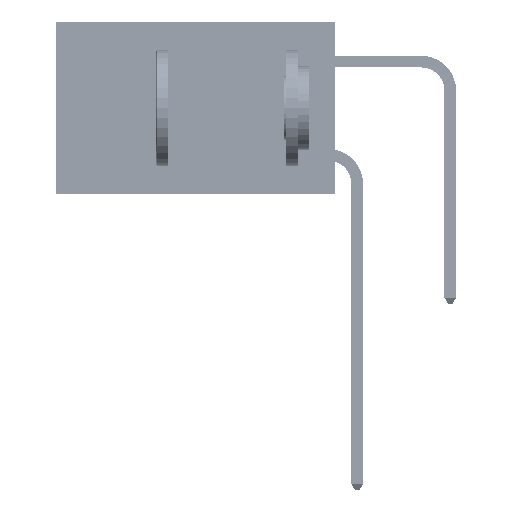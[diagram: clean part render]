
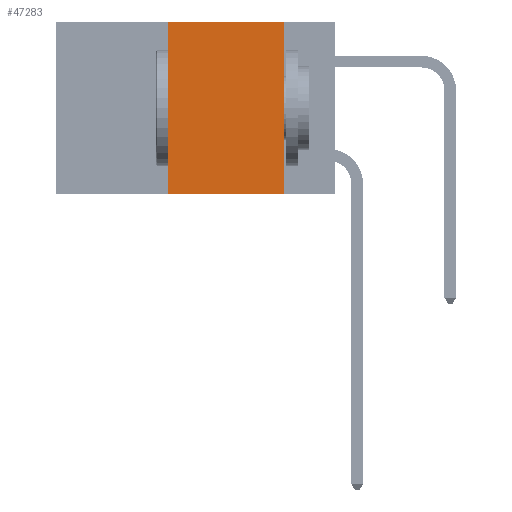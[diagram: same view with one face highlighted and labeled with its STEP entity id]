
A CAD part, left-side view. The second image highlights one B-rep face of the part: STEP entity #47283.
In plain terms, the highlighted planar face has unit normal (-1, 0, 0).
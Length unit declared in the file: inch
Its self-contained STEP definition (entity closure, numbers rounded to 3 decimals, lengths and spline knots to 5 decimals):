
#4005 = DIRECTION ( 'NONE',  ( 0., 0., -1. ) ) ;
#4142 = EDGE_CURVE ( 'NONE', #15398, #4536, #16195, .T. ) ;
#4536 = VERTEX_POINT ( 'NONE', #39910 ) ;
#6880 = ORIENTED_EDGE ( 'NONE', *, *, #33889, .F. ) ;
#7804 = LINE ( 'NONE', #27506, #16931 ) ;
#8382 = EDGE_CURVE ( 'NONE', #39591, #4536, #23125, .T. ) ;
#8922 = FACE_OUTER_BOUND ( 'NONE', #11818, .T. ) ;
#11818 = EDGE_LOOP ( 'NONE', ( #13597, #6880, #40870, #22236 ) ) ;
#11929 = CARTESIAN_POINT ( 'NONE',  ( 0., 0.11, 0. ) ) ;
#13597 = ORIENTED_EDGE ( 'NONE', *, *, #8382, .F. ) ;
#15032 = LINE ( 'NONE', #28400, #34157 ) ;
#15398 = VERTEX_POINT ( 'NONE', #15858 ) ;
#15858 = CARTESIAN_POINT ( 'NONE',  ( 0., 0.36, -0.37 ) ) ;
#16195 = LINE ( 'NONE', #22631, #35332 ) ;
#16931 = VECTOR ( 'NONE', #31310, 39.37008 ) ;
#21931 = DIRECTION ( 'NONE',  ( 0., 0., -1. ) ) ;
#22236 = ORIENTED_EDGE ( 'NONE', *, *, #4142, .T. ) ;
#22631 = CARTESIAN_POINT ( 'NONE',  ( 0., 0.6, -0.37 ) ) ;
#23125 = LINE ( 'NONE', #48547, #42202 ) ;
#23296 = PLANE ( 'NONE',  #28198 ) ;
#24350 = VERTEX_POINT ( 'NONE', #28194 ) ;
#27139 = DIRECTION ( 'NONE',  ( 1., 0., 0. ) ) ;
#27506 = CARTESIAN_POINT ( 'NONE',  ( 0., 0.36, 0. ) ) ;
#28194 = CARTESIAN_POINT ( 'NONE',  ( 0., 0.36, 0. ) ) ;
#28198 = AXIS2_PLACEMENT_3D ( 'NONE', #42284, #27139, #4005 ) ;
#28400 = CARTESIAN_POINT ( 'NONE',  ( 0., 0.6, 0. ) ) ;
#31310 = DIRECTION ( 'NONE',  ( 0., 0., 1. ) ) ;
#32241 = DIRECTION ( 'NONE',  ( 0., -1., 0. ) ) ;
#33889 = EDGE_CURVE ( 'NONE', #24350, #39591, #15032, .T. ) ;
#34157 = VECTOR ( 'NONE', #32241, 39.37008 ) ;
#35332 = VECTOR ( 'NONE', #49221, 39.37008 ) ;
#39591 = VERTEX_POINT ( 'NONE', #11929 ) ;
#39910 = CARTESIAN_POINT ( 'NONE',  ( 0., 0.11, -0.37 ) ) ;
#40183 = EDGE_CURVE ( 'NONE', #15398, #24350, #7804, .T. ) ;
#40870 = ORIENTED_EDGE ( 'NONE', *, *, #40183, .F. ) ;
#42202 = VECTOR ( 'NONE', #21931, 39.37008 ) ;
#42284 = CARTESIAN_POINT ( 'NONE',  ( 0., 0.6, 0. ) ) ;
#47283 = ADVANCED_FACE ( 'NONE', ( #8922 ), #23296, .F. ) ;
#48547 = CARTESIAN_POINT ( 'NONE',  ( 0., 0.11, 0. ) ) ;
#49221 = DIRECTION ( 'NONE',  ( 0., -1., 0. ) ) ;
